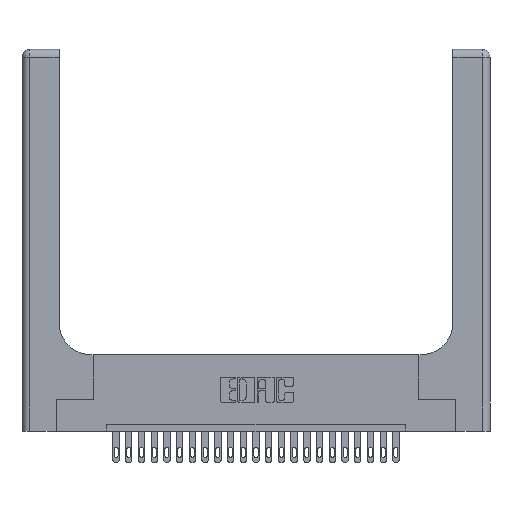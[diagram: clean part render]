
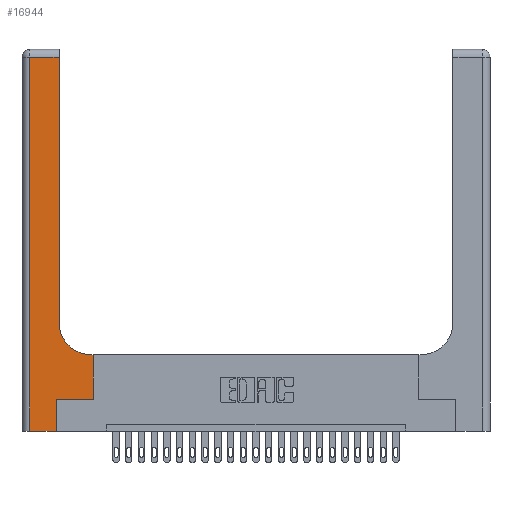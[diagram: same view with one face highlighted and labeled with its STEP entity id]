
A CAD part, top view. The second image highlights one B-rep face of the part: STEP entity #16944.
In plain terms, the highlighted planar face has unit normal (0, 0, 1).
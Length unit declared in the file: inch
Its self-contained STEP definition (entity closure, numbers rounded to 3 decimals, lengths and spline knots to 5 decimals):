
#211 = ORIENTED_EDGE ( 'NONE', *, *, #15902, .T. ) ;
#795 = EDGE_CURVE ( 'NONE', #5846, #1083, #17194, .T. ) ;
#991 = VERTEX_POINT ( 'NONE', #15126 ) ;
#1083 = VERTEX_POINT ( 'NONE', #24656 ) ;
#1116 = DIRECTION ( 'NONE',  ( 1., 0., 0. ) ) ;
#1118 = ORIENTED_EDGE ( 'NONE', *, *, #11462, .T. ) ;
#1139 = DIRECTION ( 'NONE',  ( 1., 0., 0. ) ) ;
#1344 = ORIENTED_EDGE ( 'NONE', *, *, #795, .T. ) ;
#1434 = VECTOR ( 'NONE', #24397, 39.37008 ) ;
#1504 = DIRECTION ( 'NONE',  ( 0., 1., 0. ) ) ;
#1795 = VERTEX_POINT ( 'NONE', #6764 ) ;
#2400 = CARTESIAN_POINT ( 'NONE',  ( 0.2915, 0.85, 0.37 ) ) ;
#2704 = EDGE_CURVE ( 'NONE', #1795, #17205, #14401, .T. ) ;
#2879 = VERTEX_POINT ( 'NONE', #10075 ) ;
#3366 = ORIENTED_EDGE ( 'NONE', *, *, #21094, .T. ) ;
#3415 = DIRECTION ( 'NONE',  ( 0., 0., -1. ) ) ;
#3828 = LINE ( 'NONE', #6710, #1434 ) ;
#4127 = CIRCLE ( 'NONE', #11737, 0.25 ) ;
#4525 = DIRECTION ( 'NONE',  ( 0., 1., 0. ) ) ;
#4758 = DIRECTION ( 'NONE',  ( -1., 0., 0. ) ) ;
#4791 = LINE ( 'NONE', #14206, #22602 ) ;
#5010 = ORIENTED_EDGE ( 'NONE', *, *, #23346, .T. ) ;
#5364 = DIRECTION ( 'NONE',  ( 0., 0., -1. ) ) ;
#5837 = CARTESIAN_POINT ( 'NONE',  ( 0.06, 3., 0.37 ) ) ;
#5846 = VERTEX_POINT ( 'NONE', #2400 ) ;
#6042 = CARTESIAN_POINT ( 'NONE',  ( 0.5585, 0.25, 0.37 ) ) ;
#6604 = EDGE_CURVE ( 'NONE', #20058, #5846, #4127, .T. ) ;
#6710 = CARTESIAN_POINT ( 'NONE',  ( 0., 2.94, 0.37 ) ) ;
#6764 = CARTESIAN_POINT ( 'NONE',  ( 0.06, 0., 0.37 ) ) ;
#6768 = CARTESIAN_POINT ( 'NONE',  ( 0.5585, 0.25, 0.37 ) ) ;
#7144 = LINE ( 'NONE', #8678, #16791 ) ;
#7580 = DIRECTION ( 'NONE',  ( -1., 0., 0. ) ) ;
#7751 = VECTOR ( 'NONE', #1139, 39.37008 ) ;
#8155 = VECTOR ( 'NONE', #1504, 39.37008 ) ;
#8621 = CARTESIAN_POINT ( 'NONE',  ( 0.269, 0.25, 0.37 ) ) ;
#8678 = CARTESIAN_POINT ( 'NONE',  ( 0.269, 0., 0.37 ) ) ;
#8711 = ORIENTED_EDGE ( 'NONE', *, *, #6604, .T. ) ;
#8783 = CARTESIAN_POINT ( 'NONE',  ( 0.269, 0.25, 0.37 ) ) ;
#8829 = VERTEX_POINT ( 'NONE', #8621 ) ;
#8913 = LINE ( 'NONE', #5837, #10421 ) ;
#9896 = ORIENTED_EDGE ( 'NONE', *, *, #2704, .T. ) ;
#10075 = CARTESIAN_POINT ( 'NONE',  ( 0.5585, 0.6, 0.37 ) ) ;
#10421 = VECTOR ( 'NONE', #17825, 39.37008 ) ;
#10903 = AXIS2_PLACEMENT_3D ( 'NONE', #13033, #3415, #7580 ) ;
#10955 = VECTOR ( 'NONE', #20251, 39.37008 ) ;
#11462 = EDGE_CURVE ( 'NONE', #18338, #2879, #14876, .T. ) ;
#11737 = AXIS2_PLACEMENT_3D ( 'NONE', #16935, #5364, #18878 ) ;
#13033 = CARTESIAN_POINT ( 'NONE',  ( 0., 3., 0.37 ) ) ;
#14090 = CARTESIAN_POINT ( 'NONE',  ( 0.269, 0., 0.37 ) ) ;
#14206 = CARTESIAN_POINT ( 'NONE',  ( 0.2915, 0.6, 0.37 ) ) ;
#14401 = LINE ( 'NONE', #14539, #7751 ) ;
#14539 = CARTESIAN_POINT ( 'NONE',  ( 0., 0., 0.37 ) ) ;
#14666 = VECTOR ( 'NONE', #1116, 39.37008 ) ;
#14876 = LINE ( 'NONE', #6768, #10955 ) ;
#15126 = CARTESIAN_POINT ( 'NONE',  ( 0.06, 2.94, 0.37 ) ) ;
#15902 = EDGE_CURVE ( 'NONE', #17205, #8829, #7144, .T. ) ;
#16360 = EDGE_CURVE ( 'NONE', #991, #1795, #8913, .T. ) ;
#16791 = VECTOR ( 'NONE', #4525, 39.37008 ) ;
#16858 = PLANE ( 'NONE',  #10903 ) ;
#16935 = CARTESIAN_POINT ( 'NONE',  ( 0.5415, 0.85, 0.37 ) ) ;
#16944 = ADVANCED_FACE ( 'NONE', ( #20034 ), #16858, .F. ) ;
#17067 = EDGE_LOOP ( 'NONE', ( #1344, #20351, #17430, #9896, #211, #5010, #1118, #3366, #8711 ) ) ;
#17194 = LINE ( 'NONE', #23565, #8155 ) ;
#17205 = VERTEX_POINT ( 'NONE', #14090 ) ;
#17430 = ORIENTED_EDGE ( 'NONE', *, *, #16360, .T. ) ;
#17641 = EDGE_CURVE ( 'NONE', #1083, #991, #3828, .T. ) ;
#17825 = DIRECTION ( 'NONE',  ( 0., -1., 0. ) ) ;
#18338 = VERTEX_POINT ( 'NONE', #6042 ) ;
#18720 = CARTESIAN_POINT ( 'NONE',  ( 0.5415, 0.6, 0.37 ) ) ;
#18878 = DIRECTION ( 'NONE',  ( 1., 0., 0. ) ) ;
#20034 = FACE_OUTER_BOUND ( 'NONE', #17067, .T. ) ;
#20058 = VERTEX_POINT ( 'NONE', #18720 ) ;
#20251 = DIRECTION ( 'NONE',  ( 0., 1., 0. ) ) ;
#20351 = ORIENTED_EDGE ( 'NONE', *, *, #17641, .T. ) ;
#21002 = LINE ( 'NONE', #8783, #14666 ) ;
#21094 = EDGE_CURVE ( 'NONE', #2879, #20058, #4791, .T. ) ;
#22602 = VECTOR ( 'NONE', #4758, 39.37008 ) ;
#23346 = EDGE_CURVE ( 'NONE', #8829, #18338, #21002, .T. ) ;
#23565 = CARTESIAN_POINT ( 'NONE',  ( 0.2915, 3., 0.37 ) ) ;
#24397 = DIRECTION ( 'NONE',  ( -1., 0., 0. ) ) ;
#24656 = CARTESIAN_POINT ( 'NONE',  ( 0.2915, 2.94, 0.37 ) ) ;
